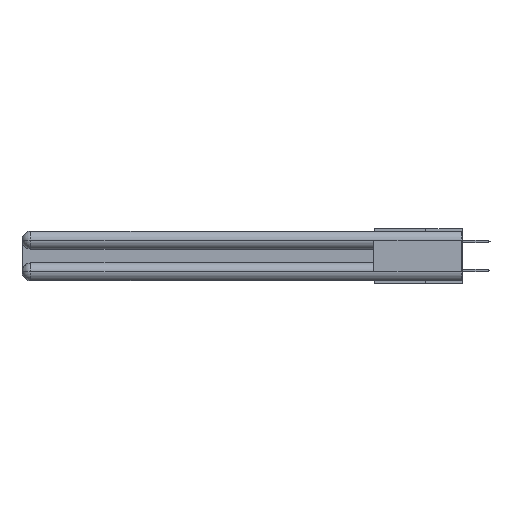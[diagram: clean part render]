
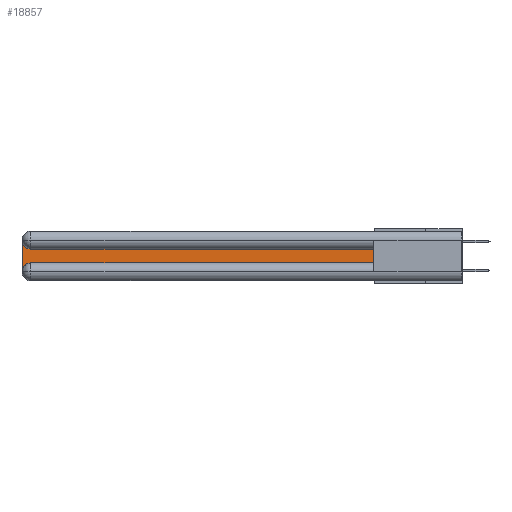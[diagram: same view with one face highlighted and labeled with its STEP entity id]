
A CAD part, left-side view. The second image highlights one B-rep face of the part: STEP entity #18857.
In plain terms, the highlighted planar face has unit normal (-1, 0, 0).
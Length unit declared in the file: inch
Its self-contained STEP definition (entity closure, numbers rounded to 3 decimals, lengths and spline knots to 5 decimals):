
#231 = EDGE_CURVE ( 'NONE', #8533, #12567, #3867, .T. ) ;
#1125 = ORIENTED_EDGE ( 'NONE', *, *, #25900, .T. ) ;
#1370 = CARTESIAN_POINT ( 'NONE',  ( 0.075, 2.94, -0.0625 ) ) ;
#1473 = DIRECTION ( 'NONE',  ( 0., 0., -1. ) ) ;
#1857 = LINE ( 'NONE', #24113, #28970 ) ;
#2387 = EDGE_CURVE ( 'NONE', #10478, #24002, #9498, .T. ) ;
#2478 = ORIENTED_EDGE ( 'NONE', *, *, #231, .T. ) ;
#2745 = AXIS2_PLACEMENT_3D ( 'NONE', #1370, #19675, #1473 ) ;
#3867 = LINE ( 'NONE', #14798, #23121 ) ;
#5751 = CIRCLE ( 'NONE', #9685, 0.06 ) ;
#5791 = VECTOR ( 'NONE', #13745, 39.37008 ) ;
#7844 = AXIS2_PLACEMENT_3D ( 'NONE', #9173, #18031, #18215 ) ;
#8533 = VERTEX_POINT ( 'NONE', #19578 ) ;
#8788 = CARTESIAN_POINT ( 'NONE',  ( 0.075, 2.94, -0.2175 ) ) ;
#9173 = CARTESIAN_POINT ( 'NONE',  ( 0.075, 3., -0.1225 ) ) ;
#9498 = LINE ( 'NONE', #11496, #26186 ) ;
#9685 = AXIS2_PLACEMENT_3D ( 'NONE', #26071, #28489, #12456 ) ;
#10478 = VERTEX_POINT ( 'NONE', #20326 ) ;
#11327 = EDGE_CURVE ( 'NONE', #28991, #10478, #25357, .T. ) ;
#11496 = CARTESIAN_POINT ( 'NONE',  ( 0.075, 0.6, -0.1225 ) ) ;
#12456 = DIRECTION ( 'NONE',  ( 0., 0., -1. ) ) ;
#12567 = VERTEX_POINT ( 'NONE', #26234 ) ;
#13487 = ORIENTED_EDGE ( 'NONE', *, *, #11327, .T. ) ;
#13745 = DIRECTION ( 'NONE',  ( 0., 0., 1. ) ) ;
#14798 = CARTESIAN_POINT ( 'NONE',  ( 0.075, 3., -0.2175 ) ) ;
#16273 = CARTESIAN_POINT ( 'NONE',  ( 0.075, 0.6, -0.2175 ) ) ;
#16891 = EDGE_CURVE ( 'NONE', #18783, #28991, #1857, .T. ) ;
#17199 = ORIENTED_EDGE ( 'NONE', *, *, #16891, .T. ) ;
#17206 = ORIENTED_EDGE ( 'NONE', *, *, #27379, .T. ) ;
#17353 = DIRECTION ( 'NONE',  ( 0., -1., 0. ) ) ;
#18031 = DIRECTION ( 'NONE',  ( 1., 0., 0. ) ) ;
#18215 = DIRECTION ( 'NONE',  ( 0., 0., -1. ) ) ;
#18783 = VERTEX_POINT ( 'NONE', #8788 ) ;
#18857 = ADVANCED_FACE ( 'NONE', ( #24177 ), #27390, .F. ) ;
#19285 = CARTESIAN_POINT ( 'NONE',  ( 0.075, 2.94, -0.1225 ) ) ;
#19578 = CARTESIAN_POINT ( 'NONE',  ( 0.075, 3., -0.0625 ) ) ;
#19675 = DIRECTION ( 'NONE',  ( 1., 0., 0. ) ) ;
#19702 = CIRCLE ( 'NONE', #2745, 0.06 ) ;
#20326 = CARTESIAN_POINT ( 'NONE',  ( 0.075, 0.6, -0.1225 ) ) ;
#20668 = ORIENTED_EDGE ( 'NONE', *, *, #2387, .T. ) ;
#20833 = DIRECTION ( 'NONE',  ( 0., 0., -1. ) ) ;
#22625 = DIRECTION ( 'NONE',  ( 0., 1., 0. ) ) ;
#23121 = VECTOR ( 'NONE', #20833, 39.37008 ) ;
#23229 = EDGE_LOOP ( 'NONE', ( #20668, #1125, #2478, #17206, #17199, #13487 ) ) ;
#24002 = VERTEX_POINT ( 'NONE', #19285 ) ;
#24113 = CARTESIAN_POINT ( 'NONE',  ( 0.075, 0.6, -0.2175 ) ) ;
#24177 = FACE_OUTER_BOUND ( 'NONE', #23229, .T. ) ;
#25357 = LINE ( 'NONE', #27507, #5791 ) ;
#25900 = EDGE_CURVE ( 'NONE', #24002, #8533, #19702, .T. ) ;
#26071 = CARTESIAN_POINT ( 'NONE',  ( 0.075, 2.94, -0.2775 ) ) ;
#26186 = VECTOR ( 'NONE', #22625, 39.37008 ) ;
#26234 = CARTESIAN_POINT ( 'NONE',  ( 0.075, 3., -0.2775 ) ) ;
#27379 = EDGE_CURVE ( 'NONE', #12567, #18783, #5751, .T. ) ;
#27390 = PLANE ( 'NONE',  #7844 ) ;
#27507 = CARTESIAN_POINT ( 'NONE',  ( 0.075, 0.6, -0.2175 ) ) ;
#28489 = DIRECTION ( 'NONE',  ( 1., 0., 0. ) ) ;
#28970 = VECTOR ( 'NONE', #17353, 39.37008 ) ;
#28991 = VERTEX_POINT ( 'NONE', #16273 ) ;
